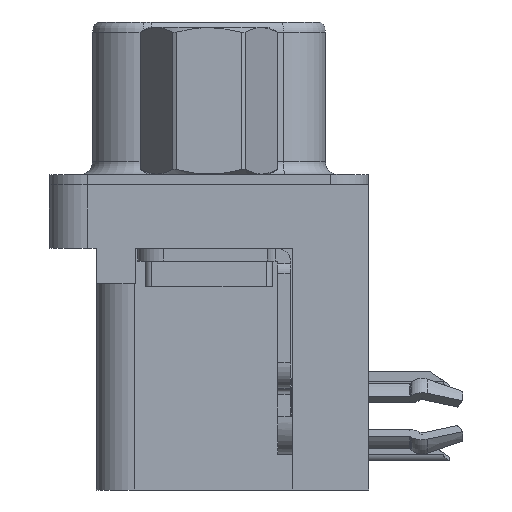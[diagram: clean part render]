
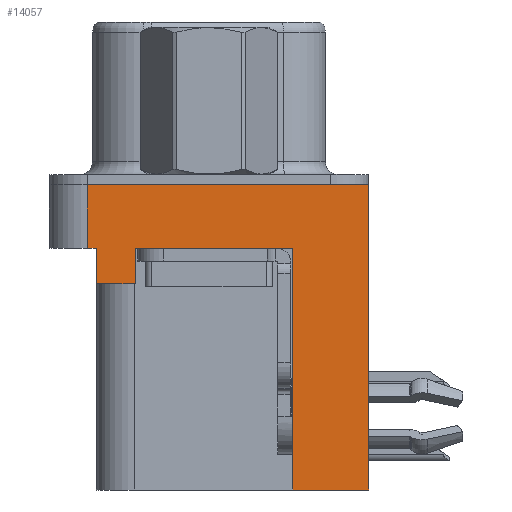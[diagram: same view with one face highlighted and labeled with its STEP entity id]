
A CAD part, left-side view. The second image highlights one B-rep face of the part: STEP entity #14057.
In plain terms, the highlighted planar face has unit normal (-1, 0, 0).
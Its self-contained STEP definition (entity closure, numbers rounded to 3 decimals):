
#963 = LINE ( 'NONE', #20115, #22462 ) ;
#964 = EDGE_CURVE ( 'NONE', #10361, #3717, #13685, .T. ) ;
#972 = ORIENTED_EDGE ( 'NONE', *, *, #4475, .F. ) ;
#1031 = DIRECTION ( 'NONE',  ( 0., 1., 0. ) ) ;
#1254 = VECTOR ( 'NONE', #24600, 1000. ) ;
#1777 = ORIENTED_EDGE ( 'NONE', *, *, #13410, .F. ) ;
#1798 = EDGE_CURVE ( 'NONE', #16605, #8275, #21438, .T. ) ;
#1974 = VECTOR ( 'NONE', #1031, 1000. ) ;
#2213 = VERTEX_POINT ( 'NONE', #4810 ) ;
#2778 = VERTEX_POINT ( 'NONE', #24016 ) ;
#3590 = VECTOR ( 'NONE', #24531, 1000. ) ;
#3717 = VERTEX_POINT ( 'NONE', #25740 ) ;
#4475 = EDGE_CURVE ( 'NONE', #21601, #10361, #13182, .T. ) ;
#4533 = DIRECTION ( 'NONE',  ( 0., 0., 1. ) ) ;
#4810 = CARTESIAN_POINT ( 'NONE',  ( -2.935, 4.425, -3.9 ) ) ;
#4872 = CARTESIAN_POINT ( 'NONE',  ( -2.935, -3.295, -12. ) ) ;
#5995 = VECTOR ( 'NONE', #9984, 1000. ) ;
#6363 = VECTOR ( 'NONE', #23308, 1000. ) ;
#6798 = CARTESIAN_POINT ( 'NONE',  ( -2.935, -3.295, -12. ) ) ;
#6858 = CARTESIAN_POINT ( 'NONE',  ( -2.935, 4.775, 0. ) ) ;
#7361 = CARTESIAN_POINT ( 'NONE',  ( -2.935, -6.275, -2.5 ) ) ;
#7600 = LINE ( 'NONE', #7361, #6363 ) ;
#7757 = EDGE_LOOP ( 'NONE', ( #1777, #10157, #10525, #13506, #13450, #22135, #15592, #24760, #972, #21317 ) ) ;
#8209 = CARTESIAN_POINT ( 'NONE',  ( -2.935, 2.895, -3.9 ) ) ;
#8275 = VERTEX_POINT ( 'NONE', #11143 ) ;
#9912 = CARTESIAN_POINT ( 'NONE',  ( -2.935, -6.275, -2.5 ) ) ;
#9914 = EDGE_CURVE ( 'NONE', #21601, #2778, #25089, .T. ) ;
#9984 = DIRECTION ( 'NONE',  ( 0., 1., 0. ) ) ;
#10157 = ORIENTED_EDGE ( 'NONE', *, *, #20749, .F. ) ;
#10361 = VERTEX_POINT ( 'NONE', #14007 ) ;
#10525 = ORIENTED_EDGE ( 'NONE', *, *, #23624, .T. ) ;
#10557 = LINE ( 'NONE', #21426, #21119 ) ;
#11087 = LINE ( 'NONE', #9912, #14737 ) ;
#11143 = CARTESIAN_POINT ( 'NONE',  ( -2.935, 2.895, -2.5 ) ) ;
#11328 = LINE ( 'NONE', #19862, #5995 ) ;
#11936 = CARTESIAN_POINT ( 'NONE',  ( -2.935, -6.275, -2.5 ) ) ;
#11955 = DIRECTION ( 'NONE',  ( 0., -1., 0. ) ) ;
#13182 = LINE ( 'NONE', #4872, #1974 ) ;
#13410 = EDGE_CURVE ( 'NONE', #22888, #2778, #963, .T. ) ;
#13450 = ORIENTED_EDGE ( 'NONE', *, *, #17698, .F. ) ;
#13506 = ORIENTED_EDGE ( 'NONE', *, *, #19080, .F. ) ;
#13685 = LINE ( 'NONE', #6798, #1254 ) ;
#14007 = CARTESIAN_POINT ( 'NONE',  ( -2.935, -3.295, -12. ) ) ;
#14057 = ADVANCED_FACE ( 'NONE', ( #21164 ), #20004, .T. ) ;
#14737 = VECTOR ( 'NONE', #15847, 1000. ) ;
#15592 = ORIENTED_EDGE ( 'NONE', *, *, #24667, .T. ) ;
#15822 = DIRECTION ( 'NONE',  ( 0., 0., 1. ) ) ;
#15847 = DIRECTION ( 'NONE',  ( 0., -1., 0. ) ) ;
#16322 = CARTESIAN_POINT ( 'NONE',  ( -2.935, -6.275, -2.5 ) ) ;
#16605 = VERTEX_POINT ( 'NONE', #19470 ) ;
#17698 = EDGE_CURVE ( 'NONE', #16605, #2213, #11328, .T. ) ;
#17711 = CARTESIAN_POINT ( 'NONE',  ( -2.935, -6.275, -12. ) ) ;
#18174 = CARTESIAN_POINT ( 'NONE',  ( -2.935, 4.775, -2.5 ) ) ;
#19080 = EDGE_CURVE ( 'NONE', #2213, #23257, #10557, .T. ) ;
#19470 = CARTESIAN_POINT ( 'NONE',  ( -2.935, 2.895, -3.9 ) ) ;
#19862 = CARTESIAN_POINT ( 'NONE',  ( -2.935, 4.425, -3.9 ) ) ;
#20004 = PLANE ( 'NONE',  #20485 ) ;
#20115 = CARTESIAN_POINT ( 'NONE',  ( -2.935, -6.275, 0. ) ) ;
#20174 = DIRECTION ( 'NONE',  ( -1., 0., 0. ) ) ;
#20420 = LINE ( 'NONE', #20467, #3590 ) ;
#20467 = CARTESIAN_POINT ( 'NONE',  ( -2.935, 4.775, -2.5 ) ) ;
#20485 = AXIS2_PLACEMENT_3D ( 'NONE', #11936, #20174, #15822 ) ;
#20589 = VERTEX_POINT ( 'NONE', #18174 ) ;
#20749 = EDGE_CURVE ( 'NONE', #20589, #22888, #20420, .T. ) ;
#21119 = VECTOR ( 'NONE', #23437, 1000. ) ;
#21164 = FACE_OUTER_BOUND ( 'NONE', #7757, .T. ) ;
#21317 = ORIENTED_EDGE ( 'NONE', *, *, #9914, .T. ) ;
#21426 = CARTESIAN_POINT ( 'NONE',  ( -2.935, 4.425, -3.9 ) ) ;
#21438 = LINE ( 'NONE', #8209, #24591 ) ;
#21601 = VERTEX_POINT ( 'NONE', #17711 ) ;
#21902 = CARTESIAN_POINT ( 'NONE',  ( -2.935, 4.425, -2.5 ) ) ;
#22135 = ORIENTED_EDGE ( 'NONE', *, *, #1798, .T. ) ;
#22145 = DIRECTION ( 'NONE',  ( 0., 0., 1. ) ) ;
#22462 = VECTOR ( 'NONE', #11955, 1000. ) ;
#22888 = VERTEX_POINT ( 'NONE', #6858 ) ;
#23257 = VERTEX_POINT ( 'NONE', #21902 ) ;
#23308 = DIRECTION ( 'NONE',  ( 0., -1., 0. ) ) ;
#23437 = DIRECTION ( 'NONE',  ( 0., 0., 1. ) ) ;
#23624 = EDGE_CURVE ( 'NONE', #20589, #23257, #7600, .T. ) ;
#24016 = CARTESIAN_POINT ( 'NONE',  ( -2.935, -6.275, 0. ) ) ;
#24531 = DIRECTION ( 'NONE',  ( 0., 0., 1. ) ) ;
#24591 = VECTOR ( 'NONE', #22145, 1000. ) ;
#24600 = DIRECTION ( 'NONE',  ( 0., 0., 1. ) ) ;
#24667 = EDGE_CURVE ( 'NONE', #8275, #3717, #11087, .T. ) ;
#24759 = VECTOR ( 'NONE', #4533, 1000. ) ;
#24760 = ORIENTED_EDGE ( 'NONE', *, *, #964, .F. ) ;
#25089 = LINE ( 'NONE', #16322, #24759 ) ;
#25740 = CARTESIAN_POINT ( 'NONE',  ( -2.935, -3.295, -2.5 ) ) ;
